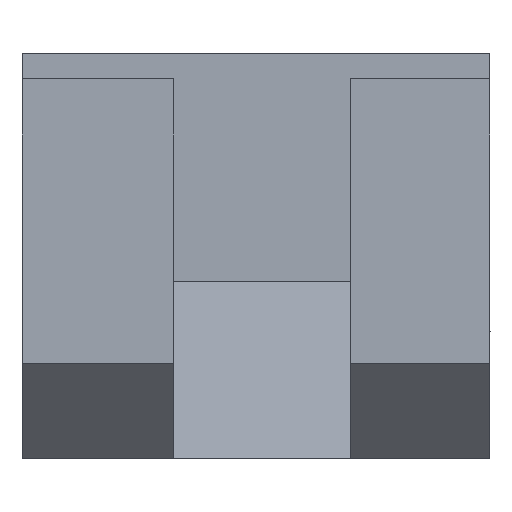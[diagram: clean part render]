
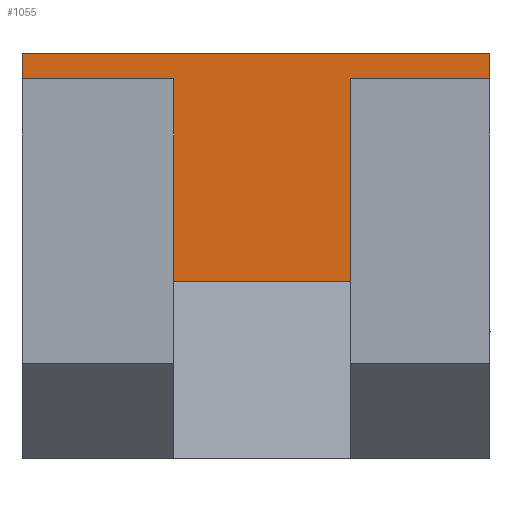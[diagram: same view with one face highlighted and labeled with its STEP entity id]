
A CAD part, left-side view. The second image highlights one B-rep face of the part: STEP entity #1055.
In plain terms, the highlighted planar face has unit normal (-1, 0, 0).
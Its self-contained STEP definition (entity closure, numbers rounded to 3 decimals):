
#55=FACE_OUTER_BOUND('',#112,.T.);
#112=EDGE_LOOP('',(#860,#861,#862,#863,#864,#865,#866));
#147=LINE('',#1438,#292);
#153=LINE('',#1451,#298);
#162=LINE('',#1469,#307);
#178=LINE('',#1499,#323);
#181=LINE('',#1505,#326);
#230=LINE('',#1605,#375);
#260=LINE('',#1661,#405);
#292=VECTOR('',#1169,10.);
#298=VECTOR('',#1179,10.);
#307=VECTOR('',#1194,10.);
#323=VECTOR('',#1212,10.);
#326=VECTOR('',#1217,10.);
#375=VECTOR('',#1292,10.);
#405=VECTOR('',#1342,10.);
#434=VERTEX_POINT('',#1431);
#436=VERTEX_POINT('',#1437);
#439=VERTEX_POINT('',#1447);
#441=VERTEX_POINT('',#1450);
#447=VERTEX_POINT('',#1468);
#462=VERTEX_POINT('',#1503);
#500=VERTEX_POINT('',#1604);
#533=EDGE_CURVE('',#434,#436,#147,.T.);
#539=EDGE_CURVE('',#441,#439,#153,.T.);
#548=EDGE_CURVE('',#447,#436,#162,.T.);
#564=EDGE_CURVE('',#441,#434,#178,.T.);
#567=EDGE_CURVE('',#462,#439,#181,.T.);
#618=EDGE_CURVE('',#500,#462,#230,.T.);
#648=EDGE_CURVE('',#500,#447,#260,.T.);
#860=ORIENTED_EDGE('',*,*,#648,.T.);
#861=ORIENTED_EDGE('',*,*,#548,.T.);
#862=ORIENTED_EDGE('',*,*,#533,.F.);
#863=ORIENTED_EDGE('',*,*,#564,.F.);
#864=ORIENTED_EDGE('',*,*,#539,.T.);
#865=ORIENTED_EDGE('',*,*,#567,.F.);
#866=ORIENTED_EDGE('',*,*,#618,.F.);
#1002=PLANE('',#1126);
#1055=ADVANCED_FACE('',(#55),#1002,.T.);
#1126=AXIS2_PLACEMENT_3D('',#1660,#1340,#1341);
#1169=DIRECTION('',(0.,1.,0.));
#1179=DIRECTION('',(0.,0.,-1.));
#1194=DIRECTION('',(0.,0.,-1.));
#1212=DIRECTION('',(0.,1.,0.));
#1217=DIRECTION('',(0.,1.,0.));
#1292=DIRECTION('',(0.,0.,-1.));
#1340=DIRECTION('center_axis',(-1.,0.,0.));
#1341=DIRECTION('ref_axis',(0.,0.,1.));
#1342=DIRECTION('',(0.,1.,0.));
#1431=CARTESIAN_POINT('',(10.5,8.25,-0.5));
#1437=CARTESIAN_POINT('',(10.5,8.25,-0.5));
#1438=CARTESIAN_POINT('',(10.5,0.,-0.5));
#1447=CARTESIAN_POINT('',(10.5,-1.,-4.));
#1450=CARTESIAN_POINT('',(10.5,-1.,-0.5));
#1451=CARTESIAN_POINT('',(10.5,-1.,-0.5));
#1468=CARTESIAN_POINT('',(10.5,8.25,4.));
#1469=CARTESIAN_POINT('',(10.5,8.25,0.));
#1499=CARTESIAN_POINT('',(10.5,0.,-0.5));
#1503=CARTESIAN_POINT('',(10.5,-1.,-4.));
#1505=CARTESIAN_POINT('',(10.5,-0.5,-4.));
#1604=CARTESIAN_POINT('',(10.5,-1.,4.));
#1605=CARTESIAN_POINT('',(10.5,-1.,-0.25));
#1660=CARTESIAN_POINT('Origin',(10.5,0.,0.));
#1661=CARTESIAN_POINT('',(10.5,0.,4.));
